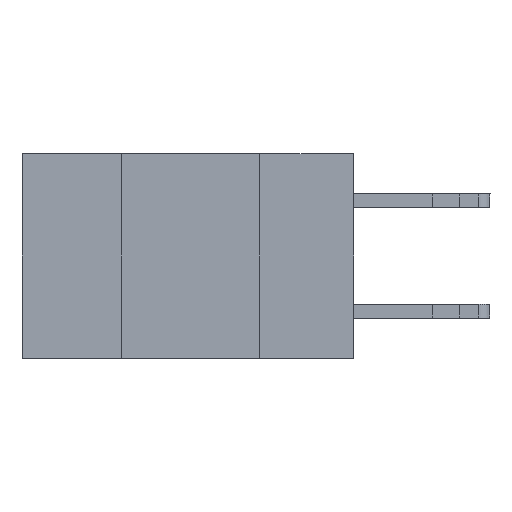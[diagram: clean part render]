
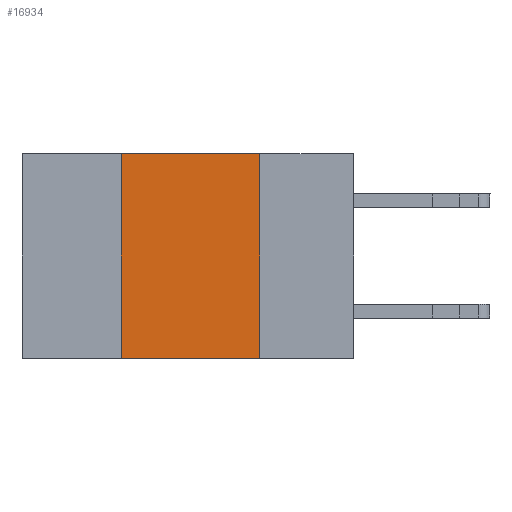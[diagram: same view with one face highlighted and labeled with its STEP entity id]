
A CAD part, left-side view. The second image highlights one B-rep face of the part: STEP entity #16934.
In plain terms, the highlighted planar face has unit normal (-1, 0, 0).
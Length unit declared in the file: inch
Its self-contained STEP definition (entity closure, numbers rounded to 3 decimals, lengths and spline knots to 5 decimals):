
#218 = DIRECTION ( 'NONE',  ( 0., -1., 0. ) ) ;
#882 = CARTESIAN_POINT ( 'NONE',  ( 0., 0.42, 0. ) ) ;
#1135 = FACE_OUTER_BOUND ( 'NONE', #9109, .T. ) ;
#1604 = VECTOR ( 'NONE', #22539, 39.37008 ) ;
#2258 = VECTOR ( 'NONE', #218, 39.37008 ) ;
#4388 = VECTOR ( 'NONE', #12292, 39.37008 ) ;
#6278 = LINE ( 'NONE', #22279, #21218 ) ;
#8375 = DIRECTION ( 'NONE',  ( 0., 0., -1. ) ) ;
#9060 = VERTEX_POINT ( 'NONE', #21251 ) ;
#9086 = AXIS2_PLACEMENT_3D ( 'NONE', #9882, #15506, #8375 ) ;
#9095 = EDGE_CURVE ( 'NONE', #16357, #9060, #19632, .T. ) ;
#9109 = EDGE_LOOP ( 'NONE', ( #10805, #15839, #14675, #19769 ) ) ;
#9557 = EDGE_CURVE ( 'NONE', #16357, #20225, #6278, .T. ) ;
#9882 = CARTESIAN_POINT ( 'NONE',  ( 0., 0.6, 0. ) ) ;
#10115 = CARTESIAN_POINT ( 'NONE',  ( 0., 0.17, 0. ) ) ;
#10805 = ORIENTED_EDGE ( 'NONE', *, *, #22592, .F. ) ;
#11763 = EDGE_CURVE ( 'NONE', #20225, #15514, #19953, .T. ) ;
#12292 = DIRECTION ( 'NONE',  ( 0., -1., 0. ) ) ;
#13855 = PLANE ( 'NONE',  #9086 ) ;
#14675 = ORIENTED_EDGE ( 'NONE', *, *, #9557, .F. ) ;
#15506 = DIRECTION ( 'NONE',  ( 1., 0., 0. ) ) ;
#15514 = VERTEX_POINT ( 'NONE', #10115 ) ;
#15548 = CARTESIAN_POINT ( 'NONE',  ( 0., 0.17, 0. ) ) ;
#15839 = ORIENTED_EDGE ( 'NONE', *, *, #11763, .F. ) ;
#16357 = VERTEX_POINT ( 'NONE', #20314 ) ;
#16561 = CARTESIAN_POINT ( 'NONE',  ( 0., 0.6, 0. ) ) ;
#16934 = ADVANCED_FACE ( 'NONE', ( #1135 ), #13855, .F. ) ;
#18463 = LINE ( 'NONE', #15548, #1604 ) ;
#19283 = CARTESIAN_POINT ( 'NONE',  ( 0., 0.6, -0.37 ) ) ;
#19632 = LINE ( 'NONE', #19283, #4388 ) ;
#19769 = ORIENTED_EDGE ( 'NONE', *, *, #9095, .T. ) ;
#19953 = LINE ( 'NONE', #16561, #2258 ) ;
#20225 = VERTEX_POINT ( 'NONE', #882 ) ;
#20314 = CARTESIAN_POINT ( 'NONE',  ( 0., 0.42, -0.37 ) ) ;
#20528 = DIRECTION ( 'NONE',  ( 0., 0., 1. ) ) ;
#21218 = VECTOR ( 'NONE', #20528, 39.37008 ) ;
#21251 = CARTESIAN_POINT ( 'NONE',  ( 0., 0.17, -0.37 ) ) ;
#22279 = CARTESIAN_POINT ( 'NONE',  ( 0., 0.42, 0. ) ) ;
#22539 = DIRECTION ( 'NONE',  ( 0., 0., -1. ) ) ;
#22592 = EDGE_CURVE ( 'NONE', #15514, #9060, #18463, .T. ) ;
